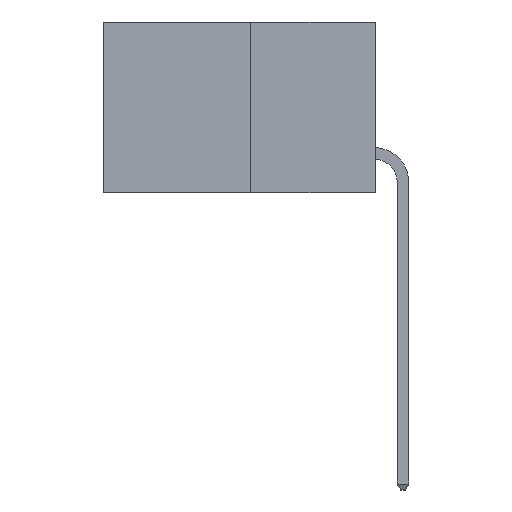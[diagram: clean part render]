
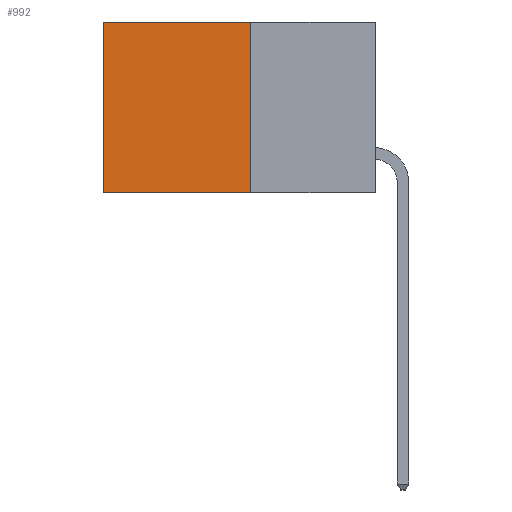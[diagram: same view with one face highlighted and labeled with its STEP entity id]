
A CAD part, left-side view. The second image highlights one B-rep face of the part: STEP entity #992.
In plain terms, the highlighted planar face has unit normal (-1, 0, 0).
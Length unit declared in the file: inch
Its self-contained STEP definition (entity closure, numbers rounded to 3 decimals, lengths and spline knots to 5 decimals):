
#111 = VECTOR ( 'NONE', #9554, 39.37008 ) ;
#332 = VERTEX_POINT ( 'NONE', #5446 ) ;
#660 = EDGE_CURVE ( 'NONE', #332, #4351, #1071, .T. ) ;
#865 = ORIENTED_EDGE ( 'NONE', *, *, #8009, .F. ) ;
#901 = CARTESIAN_POINT ( 'NONE',  ( 0.277, 0.27, -0.37 ) ) ;
#992 = ADVANCED_FACE ( 'NONE', ( #9686 ), #7330, .F. ) ;
#1071 = LINE ( 'NONE', #9010, #8956 ) ;
#1091 = LINE ( 'NONE', #8380, #7364 ) ;
#1996 = ORIENTED_EDGE ( 'NONE', *, *, #2249, .T. ) ;
#2249 = EDGE_CURVE ( 'NONE', #9238, #332, #1091, .T. ) ;
#3973 = CARTESIAN_POINT ( 'NONE',  ( 0.277, 0.27, 0. ) ) ;
#4351 = VERTEX_POINT ( 'NONE', #9997 ) ;
#4573 = LINE ( 'NONE', #901, #111 ) ;
#4802 = ORIENTED_EDGE ( 'NONE', *, *, #6653, .F. ) ;
#5069 = VECTOR ( 'NONE', #7862, 39.37008 ) ;
#5257 = CARTESIAN_POINT ( 'NONE',  ( 0.277, 0.27, -0.37 ) ) ;
#5326 = LINE ( 'NONE', #7049, #5069 ) ;
#5446 = CARTESIAN_POINT ( 'NONE',  ( 0.277, 0.59, 0. ) ) ;
#6579 = AXIS2_PLACEMENT_3D ( 'NONE', #5257, #9338, #9811 ) ;
#6653 = EDGE_CURVE ( 'NONE', #7958, #4351, #5326, .T. ) ;
#7049 = CARTESIAN_POINT ( 'NONE',  ( 0.277, 0.27, -0.37 ) ) ;
#7106 = DIRECTION ( 'NONE',  ( 0., 1., 0. ) ) ;
#7330 = PLANE ( 'NONE',  #6579 ) ;
#7364 = VECTOR ( 'NONE', #7106, 39.37008 ) ;
#7651 = ORIENTED_EDGE ( 'NONE', *, *, #660, .T. ) ;
#7691 = DIRECTION ( 'NONE',  ( 0., 0., -1. ) ) ;
#7862 = DIRECTION ( 'NONE',  ( 0., 1., 0. ) ) ;
#7958 = VERTEX_POINT ( 'NONE', #8731 ) ;
#8009 = EDGE_CURVE ( 'NONE', #9238, #7958, #4573, .T. ) ;
#8380 = CARTESIAN_POINT ( 'NONE',  ( 0.277, 0.27, 0. ) ) ;
#8731 = CARTESIAN_POINT ( 'NONE',  ( 0.277, 0.27, -0.37 ) ) ;
#8956 = VECTOR ( 'NONE', #7691, 39.37008 ) ;
#9010 = CARTESIAN_POINT ( 'NONE',  ( 0.277, 0.59, -0.37 ) ) ;
#9238 = VERTEX_POINT ( 'NONE', #3973 ) ;
#9338 = DIRECTION ( 'NONE',  ( 1., 0., 0. ) ) ;
#9554 = DIRECTION ( 'NONE',  ( 0., 0., -1. ) ) ;
#9686 = FACE_OUTER_BOUND ( 'NONE', #10120, .T. ) ;
#9811 = DIRECTION ( 'NONE',  ( 0., 0., -1. ) ) ;
#9997 = CARTESIAN_POINT ( 'NONE',  ( 0.277, 0.59, -0.37 ) ) ;
#10120 = EDGE_LOOP ( 'NONE', ( #7651, #4802, #865, #1996 ) ) ;
